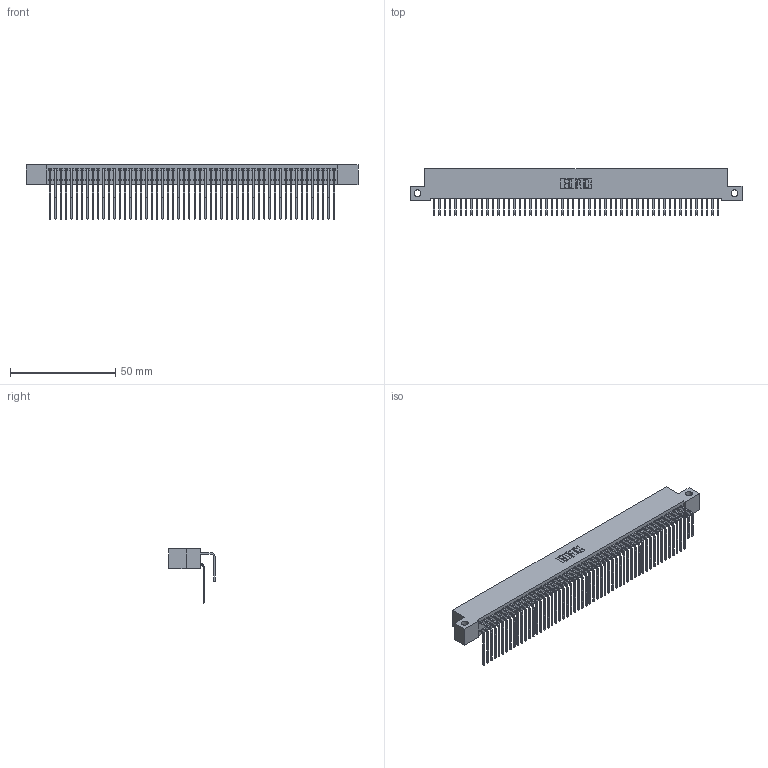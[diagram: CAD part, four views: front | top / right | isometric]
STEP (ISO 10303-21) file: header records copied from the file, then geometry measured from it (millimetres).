
FILE_DESCRIPTION (( 'STEP AP203' ), '1' );
FILE_NAME ('342-108-558-212.STEP', '2018-08-14T08:10:29', ( '' ), ( '' ), 'SwSTEP 2.0', 'SolidWorks 2016', '' );
FILE_SCHEMA (( 'CONFIG_CONTROL_DESIGN' ));
Length unit declared in the file: inch
Products named in the file (4): 342 Part_Side Mount; 345-292-001_558 559 Tail - 1; 345-292-001_558 Tail - 2; 342-108-558-212
Assembly tree (109 placements, depth 2):
  342-108-558-212
    342 Part_Side Mount
    345-292-001_558 559 Tail - 1  x54
    345-292-001_558 Tail - 2  x54
Bounding box: 157.48 x 21.91 x 25.78 mm (x, y, z)
Volume: 14755.4 mm3; surface area: 26972.4 mm2
Topology: 109 solids, 109 shells, 5942 faces, 17687 edges, 11646 vertices
Faces by surface type: plane 4170, cylinder 1772
Entity records: 34843 total; most frequent: CARTESIAN_POINT 5809, ORIENTED_EDGE 5694, DIRECTION 4923, EDGE_CURVE 2847, VECTOR 2679, LINE 2679, VERTEX_POINT 1894, AXIS2_PLACEMENT_3D 1122
